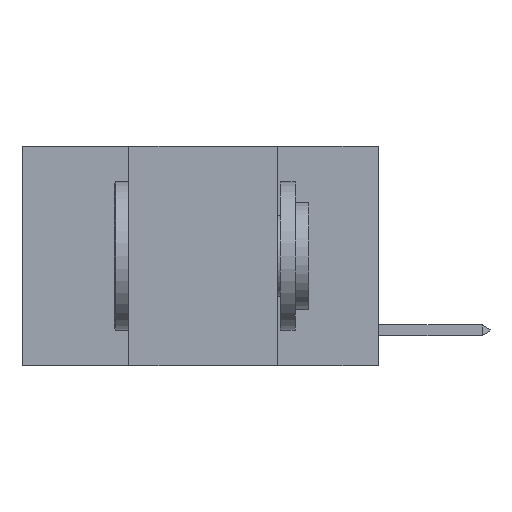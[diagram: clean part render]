
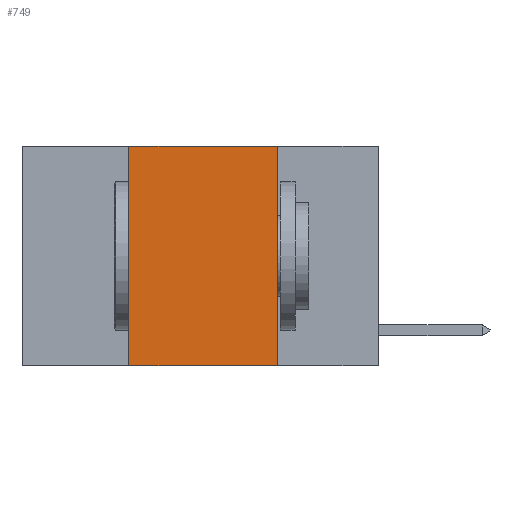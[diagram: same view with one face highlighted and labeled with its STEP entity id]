
A CAD part, left-side view. The second image highlights one B-rep face of the part: STEP entity #749.
In plain terms, the highlighted planar face has unit normal (-1, 0, 0).
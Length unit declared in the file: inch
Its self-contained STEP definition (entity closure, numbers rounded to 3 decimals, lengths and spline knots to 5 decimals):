
#62 = VECTOR ( 'NONE', #9271, 39.37008 ) ;
#749 = ADVANCED_FACE ( 'NONE', ( #19082 ), #5168, .F. ) ;
#1959 = VECTOR ( 'NONE', #3236, 39.37008 ) ;
#2519 = DIRECTION ( 'NONE',  ( 0., -1., 0. ) ) ;
#2710 = VERTEX_POINT ( 'NONE', #4089 ) ;
#3236 = DIRECTION ( 'NONE',  ( 0., 0., 1. ) ) ;
#4089 = CARTESIAN_POINT ( 'NONE',  ( 0., 0.42, 0. ) ) ;
#4673 = CARTESIAN_POINT ( 'NONE',  ( 0., 0.42, 0. ) ) ;
#4717 = VERTEX_POINT ( 'NONE', #18575 ) ;
#4800 = CARTESIAN_POINT ( 'NONE',  ( 0., 0.6, 0. ) ) ;
#5168 = PLANE ( 'NONE',  #12953 ) ;
#5806 = VERTEX_POINT ( 'NONE', #18081 ) ;
#5867 = EDGE_CURVE ( 'NONE', #14488, #5806, #17545, .T. ) ;
#6545 = ORIENTED_EDGE ( 'NONE', *, *, #5867, .F. ) ;
#7919 = EDGE_LOOP ( 'NONE', ( #6545, #11575, #8935, #12608 ) ) ;
#8935 = ORIENTED_EDGE ( 'NONE', *, *, #16628, .F. ) ;
#9271 = DIRECTION ( 'NONE',  ( 0., -1., 0. ) ) ;
#9502 = CARTESIAN_POINT ( 'NONE',  ( 0., 0.17, 0. ) ) ;
#11345 = CARTESIAN_POINT ( 'NONE',  ( 0., 0.6, 0. ) ) ;
#11575 = ORIENTED_EDGE ( 'NONE', *, *, #18239, .F. ) ;
#12264 = LINE ( 'NONE', #12458, #13246 ) ;
#12458 = CARTESIAN_POINT ( 'NONE',  ( 0., 0.6, -0.37 ) ) ;
#12608 = ORIENTED_EDGE ( 'NONE', *, *, #15231, .T. ) ;
#12945 = DIRECTION ( 'NONE',  ( 0., 0., -1. ) ) ;
#12953 = AXIS2_PLACEMENT_3D ( 'NONE', #11345, #16010, #12945 ) ;
#13246 = VECTOR ( 'NONE', #2519, 39.37008 ) ;
#13711 = LINE ( 'NONE', #4800, #62 ) ;
#14488 = VERTEX_POINT ( 'NONE', #9502 ) ;
#14495 = DIRECTION ( 'NONE',  ( 0., 0., -1. ) ) ;
#15231 = EDGE_CURVE ( 'NONE', #4717, #5806, #12264, .T. ) ;
#15725 = CARTESIAN_POINT ( 'NONE',  ( 0., 0.17, 0. ) ) ;
#15866 = VECTOR ( 'NONE', #14495, 39.37008 ) ;
#16010 = DIRECTION ( 'NONE',  ( 1., 0., 0. ) ) ;
#16628 = EDGE_CURVE ( 'NONE', #4717, #2710, #18045, .T. ) ;
#17545 = LINE ( 'NONE', #15725, #15866 ) ;
#18045 = LINE ( 'NONE', #4673, #1959 ) ;
#18081 = CARTESIAN_POINT ( 'NONE',  ( 0., 0.17, -0.37 ) ) ;
#18239 = EDGE_CURVE ( 'NONE', #2710, #14488, #13711, .T. ) ;
#18575 = CARTESIAN_POINT ( 'NONE',  ( 0., 0.42, -0.37 ) ) ;
#19082 = FACE_OUTER_BOUND ( 'NONE', #7919, .T. ) ;
